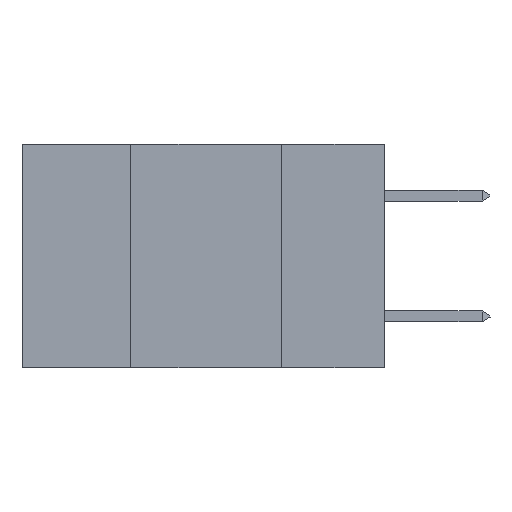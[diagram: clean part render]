
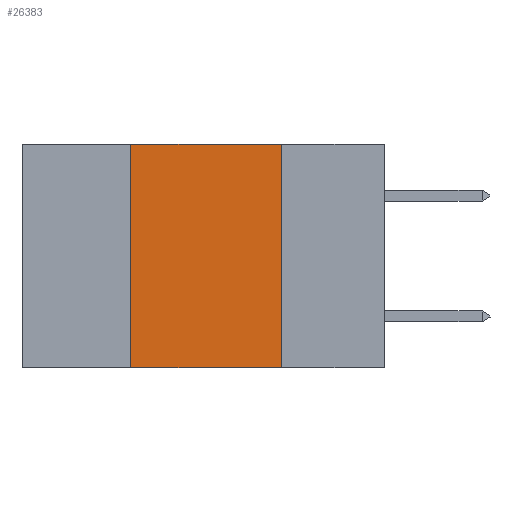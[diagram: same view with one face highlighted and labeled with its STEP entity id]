
A CAD part, left-side view. The second image highlights one B-rep face of the part: STEP entity #26383.
In plain terms, the highlighted planar face has unit normal (-1, 0, 0).
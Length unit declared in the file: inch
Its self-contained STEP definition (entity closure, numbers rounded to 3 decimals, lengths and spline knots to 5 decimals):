
#241 = LINE ( 'NONE', #6874, #17544 ) ;
#1094 = VECTOR ( 'NONE', #39324, 39.37008 ) ;
#1882 = LINE ( 'NONE', #9128, #14322 ) ;
#4479 = LINE ( 'NONE', #23989, #1094 ) ;
#5030 = VERTEX_POINT ( 'NONE', #18448 ) ;
#6874 = CARTESIAN_POINT ( 'NONE',  ( 0., 0.6, -0.37 ) ) ;
#9128 = CARTESIAN_POINT ( 'NONE',  ( 0., 0.42, 0. ) ) ;
#12517 = EDGE_CURVE ( 'NONE', #18909, #5030, #12538, .T. ) ;
#12538 = LINE ( 'NONE', #23716, #24020 ) ;
#13764 = AXIS2_PLACEMENT_3D ( 'NONE', #27695, #25090, #34050 ) ;
#14322 = VECTOR ( 'NONE', #15612, 39.37008 ) ;
#14990 = ORIENTED_EDGE ( 'NONE', *, *, #12517, .F. ) ;
#15351 = EDGE_CURVE ( 'NONE', #39414, #15776, #241, .T. ) ;
#15612 = DIRECTION ( 'NONE',  ( 0., 0., 1. ) ) ;
#15776 = VERTEX_POINT ( 'NONE', #28830 ) ;
#16779 = EDGE_CURVE ( 'NONE', #5030, #15776, #4479, .T. ) ;
#17544 = VECTOR ( 'NONE', #31622, 39.37008 ) ;
#18330 = DIRECTION ( 'NONE',  ( 0., -1., 0. ) ) ;
#18448 = CARTESIAN_POINT ( 'NONE',  ( 0., 0.17, 0. ) ) ;
#18687 = ORIENTED_EDGE ( 'NONE', *, *, #35391, .F. ) ;
#18909 = VERTEX_POINT ( 'NONE', #19834 ) ;
#19834 = CARTESIAN_POINT ( 'NONE',  ( 0., 0.42, 0. ) ) ;
#19913 = EDGE_LOOP ( 'NONE', ( #23233, #14990, #18687, #27483 ) ) ;
#23233 = ORIENTED_EDGE ( 'NONE', *, *, #16779, .F. ) ;
#23716 = CARTESIAN_POINT ( 'NONE',  ( 0., 0.6, 0. ) ) ;
#23989 = CARTESIAN_POINT ( 'NONE',  ( 0., 0.17, 0. ) ) ;
#24020 = VECTOR ( 'NONE', #18330, 39.37008 ) ;
#25090 = DIRECTION ( 'NONE',  ( 1., 0., 0. ) ) ;
#26383 = ADVANCED_FACE ( 'NONE', ( #34868 ), #33811, .F. ) ;
#27483 = ORIENTED_EDGE ( 'NONE', *, *, #15351, .T. ) ;
#27695 = CARTESIAN_POINT ( 'NONE',  ( 0., 0.6, 0. ) ) ;
#28830 = CARTESIAN_POINT ( 'NONE',  ( 0., 0.17, -0.37 ) ) ;
#31622 = DIRECTION ( 'NONE',  ( 0., -1., 0. ) ) ;
#33811 = PLANE ( 'NONE',  #13764 ) ;
#34050 = DIRECTION ( 'NONE',  ( 0., 0., -1. ) ) ;
#34868 = FACE_OUTER_BOUND ( 'NONE', #19913, .T. ) ;
#35391 = EDGE_CURVE ( 'NONE', #39414, #18909, #1882, .T. ) ;
#38733 = CARTESIAN_POINT ( 'NONE',  ( 0., 0.42, -0.37 ) ) ;
#39324 = DIRECTION ( 'NONE',  ( 0., 0., -1. ) ) ;
#39414 = VERTEX_POINT ( 'NONE', #38733 ) ;
